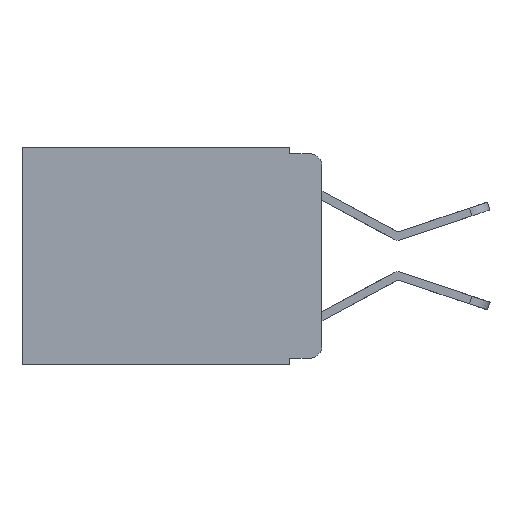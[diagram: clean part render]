
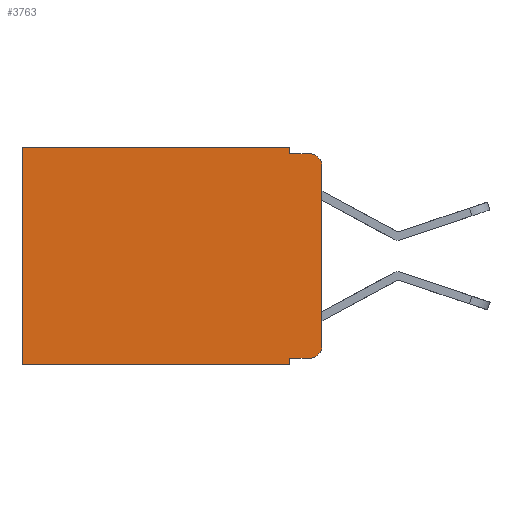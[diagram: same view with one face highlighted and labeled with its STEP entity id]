
A CAD part, left-side view. The second image highlights one B-rep face of the part: STEP entity #3763.
In plain terms, the highlighted planar face has unit normal (-1, 0, 0).
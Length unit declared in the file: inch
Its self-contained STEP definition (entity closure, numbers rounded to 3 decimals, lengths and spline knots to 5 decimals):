
#258 = CIRCLE ( 'NONE', #19898, 0.02 ) ;
#974 = CARTESIAN_POINT ( 'NONE',  ( 0.298, 0.051, 0. ) ) ;
#995 = CARTESIAN_POINT ( 'NONE',  ( 0.298, 0., 0. ) ) ;
#1103 = LINE ( 'NONE', #13768, #11800 ) ;
#1167 = ORIENTED_EDGE ( 'NONE', *, *, #12801, .T. ) ;
#1797 = LINE ( 'NONE', #18643, #3691 ) ;
#2126 = DIRECTION ( 'NONE',  ( 0., 0., -1. ) ) ;
#2258 = VERTEX_POINT ( 'NONE', #15938 ) ;
#2687 = CARTESIAN_POINT ( 'NONE',  ( 0.298, 0., 0. ) ) ;
#3084 = EDGE_CURVE ( 'NONE', #2258, #5924, #10582, .T. ) ;
#3507 = CARTESIAN_POINT ( 'NONE',  ( 0.298, 0.473, -0.343 ) ) ;
#3691 = VECTOR ( 'NONE', #7334, 39.37008 ) ;
#3733 = EDGE_CURVE ( 'NONE', #8205, #23057, #1103, .T. ) ;
#3763 = ADVANCED_FACE ( 'NONE', ( #19186 ), #22689, .F. ) ;
#4125 = VECTOR ( 'NONE', #22588, 39.37008 ) ;
#4489 = AXIS2_PLACEMENT_3D ( 'NONE', #2687, #10037, #17364 ) ;
#4515 = CARTESIAN_POINT ( 'NONE',  ( 0.298, 0., -0.03 ) ) ;
#4736 = DIRECTION ( 'NONE',  ( -1., 0., 0. ) ) ;
#4855 = CARTESIAN_POINT ( 'NONE',  ( 0.298, 0.02, -0.03 ) ) ;
#5480 = VERTEX_POINT ( 'NONE', #14291 ) ;
#5924 = VERTEX_POINT ( 'NONE', #3507 ) ;
#6468 = CARTESIAN_POINT ( 'NONE',  ( 0.298, 0.051, -0.01 ) ) ;
#6607 = CARTESIAN_POINT ( 'NONE',  ( 0.298, 0., -0.343 ) ) ;
#6712 = CARTESIAN_POINT ( 'NONE',  ( 0.298, 0.051, 0. ) ) ;
#6724 = ORIENTED_EDGE ( 'NONE', *, *, #6809, .F. ) ;
#6809 = EDGE_CURVE ( 'NONE', #5480, #2258, #15756, .T. ) ;
#7313 = LINE ( 'NONE', #15013, #7960 ) ;
#7334 = DIRECTION ( 'NONE',  ( 0., -1., 0. ) ) ;
#7960 = VECTOR ( 'NONE', #20434, 39.37008 ) ;
#8205 = VERTEX_POINT ( 'NONE', #6468 ) ;
#8375 = CARTESIAN_POINT ( 'NONE',  ( 0.298, 0.02, -0.313 ) ) ;
#8474 = DIRECTION ( 'NONE',  ( 0., 0., -1. ) ) ;
#10037 = DIRECTION ( 'NONE',  ( 1., 0., 0. ) ) ;
#10339 = ORIENTED_EDGE ( 'NONE', *, *, #21275, .F. ) ;
#10582 = LINE ( 'NONE', #6607, #12150 ) ;
#10936 = CARTESIAN_POINT ( 'NONE',  ( 0.298, 0.02, -0.01 ) ) ;
#11493 = LINE ( 'NONE', #18833, #4125 ) ;
#11800 = VECTOR ( 'NONE', #17489, 39.37008 ) ;
#11997 = EDGE_CURVE ( 'NONE', #16209, #12810, #11493, .T. ) ;
#12150 = VECTOR ( 'NONE', #13957, 39.37008 ) ;
#12180 = EDGE_CURVE ( 'NONE', #19035, #18749, #258, .T. ) ;
#12647 = ORIENTED_EDGE ( 'NONE', *, *, #3733, .F. ) ;
#12801 = EDGE_CURVE ( 'NONE', #5480, #19035, #1797, .T. ) ;
#12810 = VERTEX_POINT ( 'NONE', #22150 ) ;
#12892 = VECTOR ( 'NONE', #2126, 39.37008 ) ;
#13336 = EDGE_CURVE ( 'NONE', #16209, #8205, #7313, .T. ) ;
#13768 = CARTESIAN_POINT ( 'NONE',  ( 0.298, 0.051, -0.01 ) ) ;
#13957 = DIRECTION ( 'NONE',  ( 0., 1., 0. ) ) ;
#14291 = CARTESIAN_POINT ( 'NONE',  ( 0.298, 0.051, -0.333 ) ) ;
#15013 = CARTESIAN_POINT ( 'NONE',  ( 0.298, 0.051, 0. ) ) ;
#15388 = CARTESIAN_POINT ( 'NONE',  ( 0.298, 0.02, -0.333 ) ) ;
#15756 = LINE ( 'NONE', #6712, #17740 ) ;
#15938 = CARTESIAN_POINT ( 'NONE',  ( 0.298, 0.051, -0.343 ) ) ;
#16209 = VERTEX_POINT ( 'NONE', #974 ) ;
#16465 = ORIENTED_EDGE ( 'NONE', *, *, #20018, .T. ) ;
#16576 = CARTESIAN_POINT ( 'NONE',  ( 0.298, 0.473, 0. ) ) ;
#16788 = ORIENTED_EDGE ( 'NONE', *, *, #11997, .T. ) ;
#16832 = LINE ( 'NONE', #16576, #12892 ) ;
#16890 = EDGE_CURVE ( 'NONE', #12810, #5924, #16832, .T. ) ;
#17364 = DIRECTION ( 'NONE',  ( 0., 0., -1. ) ) ;
#17489 = DIRECTION ( 'NONE',  ( 0., -1., 0. ) ) ;
#17541 = AXIS2_PLACEMENT_3D ( 'NONE', #4855, #19550, #21232 ) ;
#17740 = VECTOR ( 'NONE', #23105, 39.37008 ) ;
#18258 = CIRCLE ( 'NONE', #17541, 0.02 ) ;
#18643 = CARTESIAN_POINT ( 'NONE',  ( 0.298, 0.051, -0.333 ) ) ;
#18749 = VERTEX_POINT ( 'NONE', #23372 ) ;
#18833 = CARTESIAN_POINT ( 'NONE',  ( 0.298, 0., 0. ) ) ;
#19035 = VERTEX_POINT ( 'NONE', #15388 ) ;
#19186 = FACE_OUTER_BOUND ( 'NONE', #19636, .T. ) ;
#19273 = ORIENTED_EDGE ( 'NONE', *, *, #16890, .T. ) ;
#19307 = ORIENTED_EDGE ( 'NONE', *, *, #3084, .F. ) ;
#19550 = DIRECTION ( 'NONE',  ( -1., 0., 0. ) ) ;
#19554 = DIRECTION ( 'NONE',  ( 0., 0., -1. ) ) ;
#19636 = EDGE_LOOP ( 'NONE', ( #10339, #16465, #12647, #21984, #16788, #19273, #19307, #6724, #1167, #21925 ) ) ;
#19898 = AXIS2_PLACEMENT_3D ( 'NONE', #8375, #4736, #8474 ) ;
#20018 = EDGE_CURVE ( 'NONE', #21250, #23057, #18258, .T. ) ;
#20434 = DIRECTION ( 'NONE',  ( 0., 0., -1. ) ) ;
#21130 = LINE ( 'NONE', #995, #21772 ) ;
#21232 = DIRECTION ( 'NONE',  ( 0., 0., -1. ) ) ;
#21250 = VERTEX_POINT ( 'NONE', #4515 ) ;
#21275 = EDGE_CURVE ( 'NONE', #21250, #18749, #21130, .T. ) ;
#21772 = VECTOR ( 'NONE', #19554, 39.37008 ) ;
#21925 = ORIENTED_EDGE ( 'NONE', *, *, #12180, .T. ) ;
#21984 = ORIENTED_EDGE ( 'NONE', *, *, #13336, .F. ) ;
#22150 = CARTESIAN_POINT ( 'NONE',  ( 0.298, 0.473, 0. ) ) ;
#22588 = DIRECTION ( 'NONE',  ( 0., 1., 0. ) ) ;
#22689 = PLANE ( 'NONE',  #4489 ) ;
#23057 = VERTEX_POINT ( 'NONE', #10936 ) ;
#23105 = DIRECTION ( 'NONE',  ( 0., 0., -1. ) ) ;
#23372 = CARTESIAN_POINT ( 'NONE',  ( 0.298, 0., -0.313 ) ) ;
